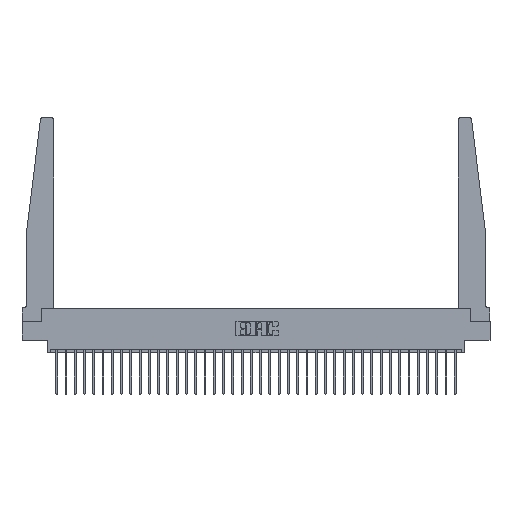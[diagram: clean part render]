
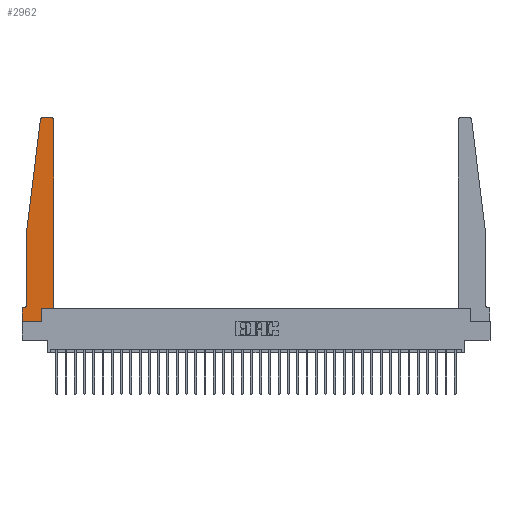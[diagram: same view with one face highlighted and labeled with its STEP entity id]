
A CAD part, top view. The second image highlights one B-rep face of the part: STEP entity #2962.
In plain terms, the highlighted planar face has unit normal (0, 0, 1).
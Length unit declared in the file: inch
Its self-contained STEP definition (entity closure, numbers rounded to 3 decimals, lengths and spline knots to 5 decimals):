
#31 = VERTEX_POINT ( 'NONE', #27491 ) ;
#251 = CARTESIAN_POINT ( 'NONE',  ( 0.2605, 0., 0.37 ) ) ;
#784 = CARTESIAN_POINT ( 'NONE',  ( 0., 0., 0.37 ) ) ;
#788 = CARTESIAN_POINT ( 'NONE',  ( 0.395, 2.72, 0.37 ) ) ;
#816 = CARTESIAN_POINT ( 'NONE',  ( 0.015, 0.2375, 0.37 ) ) ;
#1219 = LINE ( 'NONE', #784, #20974 ) ;
#1290 = CARTESIAN_POINT ( 'NONE',  ( 0.015, 0.1875, 0.37 ) ) ;
#1518 = EDGE_CURVE ( 'NONE', #2033, #7789, #4065, .T. ) ;
#2033 = VERTEX_POINT ( 'NONE', #12442 ) ;
#2126 = EDGE_CURVE ( 'NONE', #14476, #10371, #8438, .T. ) ;
#2663 = VECTOR ( 'NONE', #11330, 39.37008 ) ;
#2962 = ADVANCED_FACE ( 'NONE', ( #10009 ), #24257, .T. ) ;
#3439 = DIRECTION ( 'NONE',  ( 1., 0., 0. ) ) ;
#3468 = DIRECTION ( 'NONE',  ( -1., 0., 0. ) ) ;
#3596 = LINE ( 'NONE', #25134, #30112 ) ;
#3601 = VERTEX_POINT ( 'NONE', #29163 ) ;
#3775 = EDGE_CURVE ( 'NONE', #3601, #15846, #14733, .T. ) ;
#3832 = CARTESIAN_POINT ( 'NONE',  ( 0., 0.1875, 0.37 ) ) ;
#3918 = ORIENTED_EDGE ( 'NONE', *, *, #24460, .T. ) ;
#4065 = LINE ( 'NONE', #28300, #24521 ) ;
#5158 = LINE ( 'NONE', #24007, #30049 ) ;
#7713 = DIRECTION ( 'NONE',  ( -0.122, -0.992, 0. ) ) ;
#7789 = VERTEX_POINT ( 'NONE', #28883 ) ;
#7921 = VECTOR ( 'NONE', #14450, 39.37008 ) ;
#8438 = LINE ( 'NONE', #30639, #27284 ) ;
#8519 = AXIS2_PLACEMENT_3D ( 'NONE', #14762, #32725, #17321 ) ;
#8755 = CARTESIAN_POINT ( 'NONE',  ( 0.2605, 0.18, 0.37 ) ) ;
#8837 = ORIENTED_EDGE ( 'NONE', *, *, #32821, .T. ) ;
#9023 = DIRECTION ( 'NONE',  ( 1., 0., 0. ) ) ;
#9128 = ORIENTED_EDGE ( 'NONE', *, *, #3775, .T. ) ;
#9370 = CIRCLE ( 'NONE', #20244, 0.05 ) ;
#9871 = CARTESIAN_POINT ( 'NONE',  ( 0.24675, 2.72367, 0.37 ) ) ;
#10009 = FACE_OUTER_BOUND ( 'NONE', #33235, .T. ) ;
#10370 = CIRCLE ( 'NONE', #8519, 0.03 ) ;
#10371 = VERTEX_POINT ( 'NONE', #26657 ) ;
#11161 = EDGE_CURVE ( 'NONE', #7789, #14476, #9370, .T. ) ;
#11296 = VERTEX_POINT ( 'NONE', #11687 ) ;
#11330 = DIRECTION ( 'NONE',  ( 0., 1., 0. ) ) ;
#11687 = CARTESIAN_POINT ( 'NONE',  ( 0., 0., 0.37 ) ) ;
#11688 = ORIENTED_EDGE ( 'NONE', *, *, #30074, .T. ) ;
#12086 = VERTEX_POINT ( 'NONE', #14552 ) ;
#12092 = ORIENTED_EDGE ( 'NONE', *, *, #2126, .T. ) ;
#12223 = LINE ( 'NONE', #22985, #31095 ) ;
#12362 = DIRECTION ( 'NONE',  ( -1., 0., 0. ) ) ;
#12442 = CARTESIAN_POINT ( 'NONE',  ( 0.065, 1.25, 0.37 ) ) ;
#12775 = EDGE_CURVE ( 'NONE', #25910, #31, #3596, .T. ) ;
#12924 = DIRECTION ( 'NONE',  ( 0., -1., 0. ) ) ;
#13353 = ORIENTED_EDGE ( 'NONE', *, *, #1518, .T. ) ;
#13678 = EDGE_CURVE ( 'NONE', #10371, #11296, #5158, .T. ) ;
#13707 = EDGE_CURVE ( 'NONE', #23257, #12086, #16373, .T. ) ;
#13799 = DIRECTION ( 'NONE',  ( 0., -1., 0. ) ) ;
#13877 = ORIENTED_EDGE ( 'NONE', *, *, #31555, .T. ) ;
#14450 = DIRECTION ( 'NONE',  ( 0., 1., 0. ) ) ;
#14476 = VERTEX_POINT ( 'NONE', #1290 ) ;
#14552 = CARTESIAN_POINT ( 'NONE',  ( 0.2605, 0.18, 0.37 ) ) ;
#14733 = LINE ( 'NONE', #27116, #7921 ) ;
#14762 = CARTESIAN_POINT ( 'NONE',  ( 0.27653, 2.72, 0.37 ) ) ;
#15521 = ORIENTED_EDGE ( 'NONE', *, *, #13678, .T. ) ;
#15846 = VERTEX_POINT ( 'NONE', #30034 ) ;
#16373 = LINE ( 'NONE', #8755, #2663 ) ;
#17140 = ORIENTED_EDGE ( 'NONE', *, *, #12775, .T. ) ;
#17321 = DIRECTION ( 'NONE',  ( 1., 0., 0. ) ) ;
#18047 = ORIENTED_EDGE ( 'NONE', *, *, #26201, .T. ) ;
#18839 = DIRECTION ( 'NONE',  ( 0., 0., 1. ) ) ;
#18865 = DIRECTION ( 'NONE',  ( 0., 0., -1. ) ) ;
#19051 = VERTEX_POINT ( 'NONE', #9871 ) ;
#19271 = VECTOR ( 'NONE', #30093, 39.37008 ) ;
#19663 = AXIS2_PLACEMENT_3D ( 'NONE', #788, #18839, #3439 ) ;
#20068 = LINE ( 'NONE', #27493, #19271 ) ;
#20244 = AXIS2_PLACEMENT_3D ( 'NONE', #816, #18865, #3468 ) ;
#20974 = VECTOR ( 'NONE', #21416, 39.37008 ) ;
#21416 = DIRECTION ( 'NONE',  ( 1., 0., 0. ) ) ;
#22985 = CARTESIAN_POINT ( 'NONE',  ( 0.065, 1.25, 0.37 ) ) ;
#23257 = VERTEX_POINT ( 'NONE', #251 ) ;
#23773 = CIRCLE ( 'NONE', #19663, 0.03 ) ;
#24007 = CARTESIAN_POINT ( 'NONE',  ( 0., 0., 0.37 ) ) ;
#24257 = PLANE ( 'NONE',  #33243 ) ;
#24355 = DIRECTION ( 'NONE',  ( 0., 0., 1. ) ) ;
#24460 = EDGE_CURVE ( 'NONE', #19051, #2033, #12223, .T. ) ;
#24521 = VECTOR ( 'NONE', #12924, 39.37008 ) ;
#24633 = ORIENTED_EDGE ( 'NONE', *, *, #11161, .T. ) ;
#25134 = CARTESIAN_POINT ( 'NONE',  ( 0.25, 2.75, 0.37 ) ) ;
#25910 = VERTEX_POINT ( 'NONE', #31993 ) ;
#26201 = EDGE_CURVE ( 'NONE', #15846, #25910, #23773, .T. ) ;
#26657 = CARTESIAN_POINT ( 'NONE',  ( 0., 0.1875, 0.37 ) ) ;
#27116 = CARTESIAN_POINT ( 'NONE',  ( 0.425, 0.18, 0.37 ) ) ;
#27284 = VECTOR ( 'NONE', #33213, 39.37008 ) ;
#27491 = CARTESIAN_POINT ( 'NONE',  ( 0.27653, 2.75, 0.37 ) ) ;
#27493 = CARTESIAN_POINT ( 'NONE',  ( 0.425, 0.18, 0.37 ) ) ;
#28300 = CARTESIAN_POINT ( 'NONE',  ( 0.065, 1.25, 0.37 ) ) ;
#28883 = CARTESIAN_POINT ( 'NONE',  ( 0.065, 0.2375, 0.37 ) ) ;
#29163 = CARTESIAN_POINT ( 'NONE',  ( 0.425, 0.18, 0.37 ) ) ;
#29559 = ORIENTED_EDGE ( 'NONE', *, *, #13707, .T. ) ;
#30034 = CARTESIAN_POINT ( 'NONE',  ( 0.425, 2.72, 0.37 ) ) ;
#30049 = VECTOR ( 'NONE', #13799, 39.37008 ) ;
#30074 = EDGE_CURVE ( 'NONE', #11296, #23257, #1219, .T. ) ;
#30093 = DIRECTION ( 'NONE',  ( 1., 0., 0. ) ) ;
#30112 = VECTOR ( 'NONE', #12362, 39.37008 ) ;
#30639 = CARTESIAN_POINT ( 'NONE',  ( 0.065, 0.1875, 0.37 ) ) ;
#31095 = VECTOR ( 'NONE', #7713, 39.37008 ) ;
#31555 = EDGE_CURVE ( 'NONE', #12086, #3601, #20068, .T. ) ;
#31993 = CARTESIAN_POINT ( 'NONE',  ( 0.395, 2.75, 0.37 ) ) ;
#32725 = DIRECTION ( 'NONE',  ( 0., 0., 1. ) ) ;
#32821 = EDGE_CURVE ( 'NONE', #31, #19051, #10370, .T. ) ;
#33213 = DIRECTION ( 'NONE',  ( -1., 0., 0. ) ) ;
#33235 = EDGE_LOOP ( 'NONE', ( #17140, #8837, #3918, #13353, #24633, #12092, #15521, #11688, #29559, #13877, #9128, #18047 ) ) ;
#33243 = AXIS2_PLACEMENT_3D ( 'NONE', #3832, #24355, #9023 ) ;
